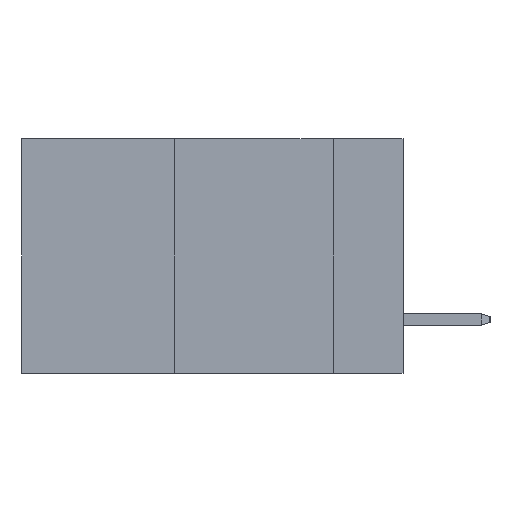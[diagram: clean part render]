
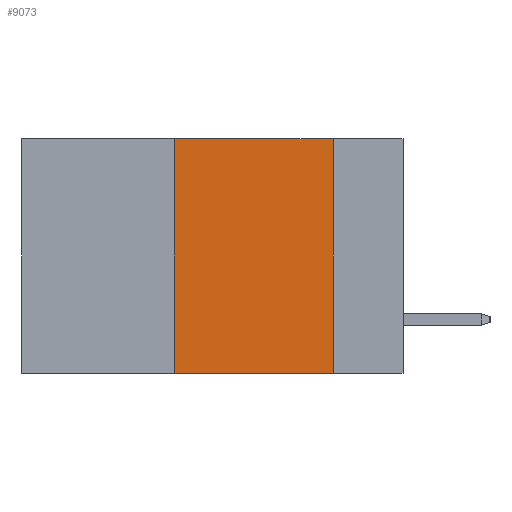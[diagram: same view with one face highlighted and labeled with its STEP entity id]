
A CAD part, left-side view. The second image highlights one B-rep face of the part: STEP entity #9073.
In plain terms, the highlighted planar face has unit normal (-1, 0, 0).
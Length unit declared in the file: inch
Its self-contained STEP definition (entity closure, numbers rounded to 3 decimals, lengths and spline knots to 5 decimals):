
#644 = VECTOR ( 'NONE', #5045, 39.37008 ) ;
#649 = PLANE ( 'NONE',  #5921 ) ;
#701 = CARTESIAN_POINT ( 'NONE',  ( 0., 0.11, 0. ) ) ;
#738 = VERTEX_POINT ( 'NONE', #6122 ) ;
#804 = CARTESIAN_POINT ( 'NONE',  ( 0., 0.6, 0. ) ) ;
#1632 = CARTESIAN_POINT ( 'NONE',  ( 0., 0.36, 0. ) ) ;
#1747 = ORIENTED_EDGE ( 'NONE', *, *, #2847, .T. ) ;
#1855 = DIRECTION ( 'NONE',  ( 0., 0., 1. ) ) ;
#2007 = CARTESIAN_POINT ( 'NONE',  ( 0., 0.6, -0.37 ) ) ;
#2801 = EDGE_CURVE ( 'NONE', #8103, #738, #12556, .T. ) ;
#2842 = DIRECTION ( 'NONE',  ( 0., -1., 0. ) ) ;
#2847 = EDGE_CURVE ( 'NONE', #6896, #738, #8459, .T. ) ;
#2848 = CARTESIAN_POINT ( 'NONE',  ( 0., 0.36, -0.37 ) ) ;
#3867 = DIRECTION ( 'NONE',  ( 0., 0., -1. ) ) ;
#5045 = DIRECTION ( 'NONE',  ( 0., 0., -1. ) ) ;
#5092 = DIRECTION ( 'NONE',  ( 0., -1., 0. ) ) ;
#5921 = AXIS2_PLACEMENT_3D ( 'NONE', #11045, #12446, #3867 ) ;
#6122 = CARTESIAN_POINT ( 'NONE',  ( 0., 0.11, -0.37 ) ) ;
#6501 = ORIENTED_EDGE ( 'NONE', *, *, #12247, .F. ) ;
#6896 = VERTEX_POINT ( 'NONE', #2848 ) ;
#7139 = ORIENTED_EDGE ( 'NONE', *, *, #7356, .F. ) ;
#7356 = EDGE_CURVE ( 'NONE', #6896, #11665, #13741, .T. ) ;
#8103 = VERTEX_POINT ( 'NONE', #701 ) ;
#8161 = EDGE_LOOP ( 'NONE', ( #11472, #6501, #7139, #1747 ) ) ;
#8459 = LINE ( 'NONE', #2007, #10740 ) ;
#9073 = ADVANCED_FACE ( 'NONE', ( #10257 ), #649, .F. ) ;
#10123 = VECTOR ( 'NONE', #1855, 39.37008 ) ;
#10257 = FACE_OUTER_BOUND ( 'NONE', #8161, .T. ) ;
#10416 = LINE ( 'NONE', #804, #13210 ) ;
#10639 = CARTESIAN_POINT ( 'NONE',  ( 0., 0.36, 0. ) ) ;
#10740 = VECTOR ( 'NONE', #2842, 39.37008 ) ;
#11045 = CARTESIAN_POINT ( 'NONE',  ( 0., 0.6, 0. ) ) ;
#11472 = ORIENTED_EDGE ( 'NONE', *, *, #2801, .F. ) ;
#11635 = CARTESIAN_POINT ( 'NONE',  ( 0., 0.11, 0. ) ) ;
#11665 = VERTEX_POINT ( 'NONE', #1632 ) ;
#12247 = EDGE_CURVE ( 'NONE', #11665, #8103, #10416, .T. ) ;
#12446 = DIRECTION ( 'NONE',  ( 1., 0., 0. ) ) ;
#12556 = LINE ( 'NONE', #11635, #644 ) ;
#13210 = VECTOR ( 'NONE', #5092, 39.37008 ) ;
#13741 = LINE ( 'NONE', #10639, #10123 ) ;
